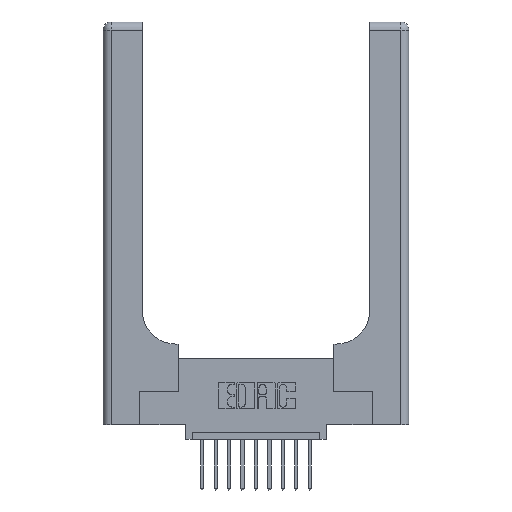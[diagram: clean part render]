
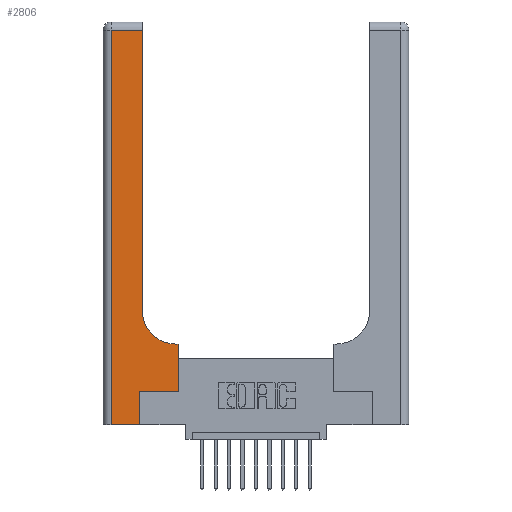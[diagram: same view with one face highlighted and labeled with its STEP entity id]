
A CAD part, top view. The second image highlights one B-rep face of the part: STEP entity #2806.
In plain terms, the highlighted planar face has unit normal (0, 0, 1).
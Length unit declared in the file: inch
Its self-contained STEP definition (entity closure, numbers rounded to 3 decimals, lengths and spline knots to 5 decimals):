
#223 = VECTOR ( 'NONE', #2797, 39.37008 ) ;
#419 = VERTEX_POINT ( 'NONE', #1974 ) ;
#594 = ORIENTED_EDGE ( 'NONE', *, *, #6927, .T. ) ;
#789 = VECTOR ( 'NONE', #12707, 39.37008 ) ;
#791 = ORIENTED_EDGE ( 'NONE', *, *, #11120, .T. ) ;
#1707 = CARTESIAN_POINT ( 'NONE',  ( 0.06, 0., 0.37 ) ) ;
#1939 = CARTESIAN_POINT ( 'NONE',  ( 0.2915, 3., 0.37 ) ) ;
#1974 = CARTESIAN_POINT ( 'NONE',  ( 0.06, 2.94, 0.37 ) ) ;
#2354 = ORIENTED_EDGE ( 'NONE', *, *, #6518, .T. ) ;
#2473 = CARTESIAN_POINT ( 'NONE',  ( 0.269, 0., 0.37 ) ) ;
#2698 = CARTESIAN_POINT ( 'NONE',  ( 0.269, 0.25, 0.37 ) ) ;
#2797 = DIRECTION ( 'NONE',  ( 0., 1., 0. ) ) ;
#2806 = ADVANCED_FACE ( 'NONE', ( #5528 ), #12969, .F. ) ;
#3312 = VERTEX_POINT ( 'NONE', #12325 ) ;
#4060 = CARTESIAN_POINT ( 'NONE',  ( 0.5585, 0.6, 0.37 ) ) ;
#4606 = DIRECTION ( 'NONE',  ( 0., 1., 0. ) ) ;
#4681 = DIRECTION ( 'NONE',  ( -1., 0., 0. ) ) ;
#5023 = VERTEX_POINT ( 'NONE', #13176 ) ;
#5328 = ORIENTED_EDGE ( 'NONE', *, *, #13077, .T. ) ;
#5528 = FACE_OUTER_BOUND ( 'NONE', #15349, .T. ) ;
#5782 = ORIENTED_EDGE ( 'NONE', *, *, #7138, .T. ) ;
#5788 = LINE ( 'NONE', #10256, #789 ) ;
#5880 = DIRECTION ( 'NONE',  ( -1., 0., 0. ) ) ;
#6028 = CARTESIAN_POINT ( 'NONE',  ( 0.5415, 0.85, 0.37 ) ) ;
#6269 = VECTOR ( 'NONE', #5880, 39.37008 ) ;
#6288 = CIRCLE ( 'NONE', #10231, 0.25 ) ;
#6375 = VERTEX_POINT ( 'NONE', #13314 ) ;
#6508 = EDGE_CURVE ( 'NONE', #6375, #419, #15576, .T. ) ;
#6518 = EDGE_CURVE ( 'NONE', #419, #7408, #14403, .T. ) ;
#6612 = CARTESIAN_POINT ( 'NONE',  ( 0., 3., 0.37 ) ) ;
#6927 = EDGE_CURVE ( 'NONE', #3312, #15011, #9206, .T. ) ;
#7138 = EDGE_CURVE ( 'NONE', #7408, #12258, #5788, .T. ) ;
#7408 = VERTEX_POINT ( 'NONE', #1707 ) ;
#7571 = VECTOR ( 'NONE', #12678, 39.37008 ) ;
#7719 = ORIENTED_EDGE ( 'NONE', *, *, #12838, .T. ) ;
#8010 = VERTEX_POINT ( 'NONE', #12172 ) ;
#8016 = EDGE_CURVE ( 'NONE', #13424, #6375, #8687, .T. ) ;
#8534 = DIRECTION ( 'NONE',  ( 1., 0., 0. ) ) ;
#8687 = LINE ( 'NONE', #1939, #223 ) ;
#9206 = LINE ( 'NONE', #9661, #15377 ) ;
#9661 = CARTESIAN_POINT ( 'NONE',  ( 0.5585, 0.25, 0.37 ) ) ;
#9711 = ORIENTED_EDGE ( 'NONE', *, *, #6508, .T. ) ;
#10192 = VECTOR ( 'NONE', #14990, 39.37008 ) ;
#10231 = AXIS2_PLACEMENT_3D ( 'NONE', #6028, #11153, #8534 ) ;
#10256 = CARTESIAN_POINT ( 'NONE',  ( 0., 0., 0.37 ) ) ;
#10353 = DIRECTION ( 'NONE',  ( 0., 0., -1. ) ) ;
#10946 = LINE ( 'NONE', #2473, #7571 ) ;
#11083 = CARTESIAN_POINT ( 'NONE',  ( 0.06, 3., 0.37 ) ) ;
#11120 = EDGE_CURVE ( 'NONE', #8010, #3312, #16516, .T. ) ;
#11153 = DIRECTION ( 'NONE',  ( 0., 0., -1. ) ) ;
#11343 = EDGE_CURVE ( 'NONE', #12258, #8010, #10946, .T. ) ;
#11557 = DIRECTION ( 'NONE',  ( -1., 0., 0. ) ) ;
#11698 = CARTESIAN_POINT ( 'NONE',  ( 0.2915, 0.85, 0.37 ) ) ;
#12172 = CARTESIAN_POINT ( 'NONE',  ( 0.269, 0.25, 0.37 ) ) ;
#12258 = VERTEX_POINT ( 'NONE', #13508 ) ;
#12325 = CARTESIAN_POINT ( 'NONE',  ( 0.5585, 0.25, 0.37 ) ) ;
#12375 = CARTESIAN_POINT ( 'NONE',  ( 0.2915, 0.6, 0.37 ) ) ;
#12417 = CARTESIAN_POINT ( 'NONE',  ( 0., 2.94, 0.37 ) ) ;
#12678 = DIRECTION ( 'NONE',  ( 0., 1., 0. ) ) ;
#12707 = DIRECTION ( 'NONE',  ( 1., 0., 0. ) ) ;
#12838 = EDGE_CURVE ( 'NONE', #5023, #13424, #6288, .T. ) ;
#12924 = ORIENTED_EDGE ( 'NONE', *, *, #11343, .T. ) ;
#12969 = PLANE ( 'NONE',  #13800 ) ;
#13077 = EDGE_CURVE ( 'NONE', #15011, #5023, #16439, .T. ) ;
#13176 = CARTESIAN_POINT ( 'NONE',  ( 0.5415, 0.6, 0.37 ) ) ;
#13314 = CARTESIAN_POINT ( 'NONE',  ( 0.2915, 2.94, 0.37 ) ) ;
#13424 = VERTEX_POINT ( 'NONE', #11698 ) ;
#13508 = CARTESIAN_POINT ( 'NONE',  ( 0.269, 0., 0.37 ) ) ;
#13800 = AXIS2_PLACEMENT_3D ( 'NONE', #6612, #10353, #11557 ) ;
#13999 = VECTOR ( 'NONE', #4681, 39.37008 ) ;
#14403 = LINE ( 'NONE', #11083, #10192 ) ;
#14990 = DIRECTION ( 'NONE',  ( 0., -1., 0. ) ) ;
#15011 = VERTEX_POINT ( 'NONE', #4060 ) ;
#15328 = DIRECTION ( 'NONE',  ( 1., 0., 0. ) ) ;
#15349 = EDGE_LOOP ( 'NONE', ( #16563, #9711, #2354, #5782, #12924, #791, #594, #5328, #7719 ) ) ;
#15377 = VECTOR ( 'NONE', #4606, 39.37008 ) ;
#15576 = LINE ( 'NONE', #12417, #13999 ) ;
#16315 = VECTOR ( 'NONE', #15328, 39.37008 ) ;
#16439 = LINE ( 'NONE', #12375, #6269 ) ;
#16516 = LINE ( 'NONE', #2698, #16315 ) ;
#16563 = ORIENTED_EDGE ( 'NONE', *, *, #8016, .T. ) ;
